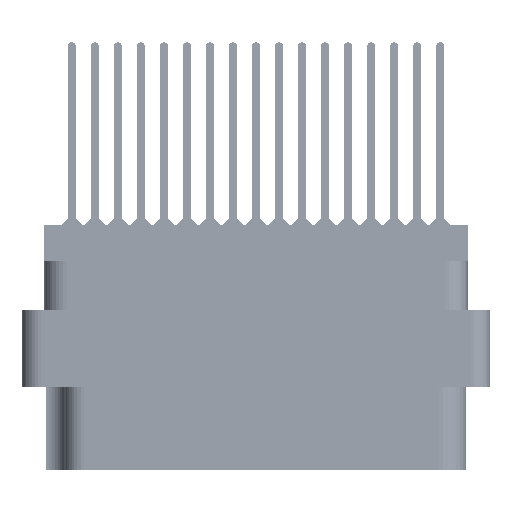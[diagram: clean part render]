
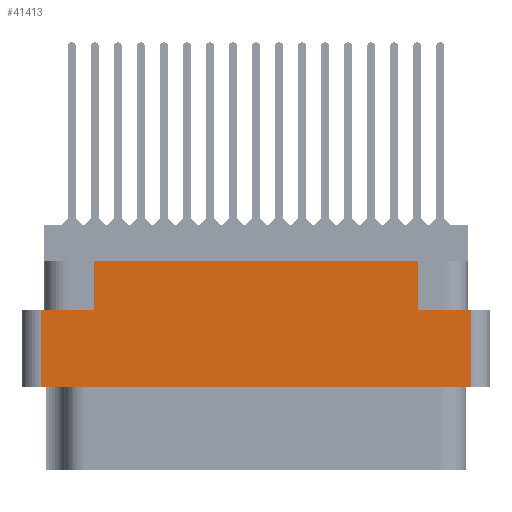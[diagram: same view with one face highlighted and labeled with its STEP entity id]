
A CAD part, left-side view. The second image highlights one B-rep face of the part: STEP entity #41413.
In plain terms, the highlighted planar face has unit normal (-1, 0, 0).
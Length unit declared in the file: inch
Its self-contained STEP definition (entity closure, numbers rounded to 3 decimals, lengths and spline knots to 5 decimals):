
#4939 = DIRECTION ( 'NONE',  ( 0., 0., 1. ) ) ;
#6147 = VECTOR ( 'NONE', #4939, 39.37008 ) ;
#7353 = DIRECTION ( 'NONE',  ( 0., -1., 0. ) ) ;
#7427 = CARTESIAN_POINT ( 'NONE',  ( -1.375, 0.7625, -0.117 ) ) ;
#7604 = CARTESIAN_POINT ( 'NONE',  ( -1.375, -0.7005, -0.798 ) ) ;
#7674 = CARTESIAN_POINT ( 'NONE',  ( -1.375, 0., -0.277 ) ) ;
#8654 = LINE ( 'NONE', #7604, #18909 ) ;
#11909 = VECTOR ( 'NONE', #84373, 39.37008 ) ;
#12399 = ORIENTED_EDGE ( 'NONE', *, *, #70454, .F. ) ;
#13224 = EDGE_CURVE ( 'NONE', #89813, #68162, #82296, .T. ) ;
#13752 = EDGE_CURVE ( 'NONE', #39072, #81822, #75394, .T. ) ;
#18715 = ORIENTED_EDGE ( 'NONE', *, *, #13752, .F. ) ;
#18909 = VECTOR ( 'NONE', #22811, 39.37008 ) ;
#20051 = LINE ( 'NONE', #7427, #66583 ) ;
#22471 = DIRECTION ( 'NONE',  ( 0., 0., 1. ) ) ;
#22811 = DIRECTION ( 'NONE',  ( 0., 0., 1. ) ) ;
#23578 = ORIENTED_EDGE ( 'NONE', *, *, #89172, .F. ) ;
#24195 = ORIENTED_EDGE ( 'NONE', *, *, #91789, .T. ) ;
#27021 = VERTEX_POINT ( 'NONE', #82789 ) ;
#27518 = CARTESIAN_POINT ( 'NONE',  ( -1.375, 0.5285, -0.117 ) ) ;
#28027 = DIRECTION ( 'NONE',  ( -1., 0., 0. ) ) ;
#29337 = LINE ( 'NONE', #7674, #58841 ) ;
#33437 = VECTOR ( 'NONE', #79629, 39.37008 ) ;
#35341 = ORIENTED_EDGE ( 'NONE', *, *, #47945, .F. ) ;
#38995 = AXIS2_PLACEMENT_3D ( 'NONE', #92511, #28027, #48742 ) ;
#39009 = VECTOR ( 'NONE', #22471, 39.37008 ) ;
#39072 = VERTEX_POINT ( 'NONE', #85633 ) ;
#40342 = EDGE_CURVE ( 'NONE', #90785, #66365, #8654, .T. ) ;
#41413 = ADVANCED_FACE ( 'NONE', ( #49441 ), #56936, .T. ) ;
#47945 = EDGE_CURVE ( 'NONE', #90785, #68162, #82249, .T. ) ;
#48142 = LINE ( 'NONE', #65962, #39009 ) ;
#48742 = DIRECTION ( 'NONE',  ( 0., 0., 1. ) ) ;
#49441 = FACE_OUTER_BOUND ( 'NONE', #58617, .T. ) ;
#50469 = CARTESIAN_POINT ( 'NONE',  ( -1.375, 0., -0.529 ) ) ;
#56936 = PLANE ( 'NONE',  #38995 ) ;
#57621 = DIRECTION ( 'NONE',  ( 0., -1., 0. ) ) ;
#58617 = EDGE_LOOP ( 'NONE', ( #12399, #67924, #35341, #63581, #23578, #24195, #81242, #18715 ) ) ;
#58841 = VECTOR ( 'NONE', #7353, 39.37008 ) ;
#60055 = VERTEX_POINT ( 'NONE', #82820 ) ;
#61854 = LINE ( 'NONE', #92574, #89124 ) ;
#63581 = ORIENTED_EDGE ( 'NONE', *, *, #40342, .T. ) ;
#65962 = CARTESIAN_POINT ( 'NONE',  ( -1.375, -0.5285, -0.277 ) ) ;
#66365 = VERTEX_POINT ( 'NONE', #68093 ) ;
#66583 = VECTOR ( 'NONE', #57621, 39.37008 ) ;
#67924 = ORIENTED_EDGE ( 'NONE', *, *, #13224, .T. ) ;
#68093 = CARTESIAN_POINT ( 'NONE',  ( -1.375, -0.7005, -0.277 ) ) ;
#68162 = VERTEX_POINT ( 'NONE', #82599 ) ;
#69620 = EDGE_CURVE ( 'NONE', #81822, #27021, #20051, .T. ) ;
#70257 = CARTESIAN_POINT ( 'NONE',  ( -1.375, -0.7005, -0.529 ) ) ;
#70454 = EDGE_CURVE ( 'NONE', #89813, #39072, #61854, .T. ) ;
#75394 = LINE ( 'NONE', #91957, #6147 ) ;
#77045 = CARTESIAN_POINT ( 'NONE',  ( -1.375, 0.7005, -0.798 ) ) ;
#79629 = DIRECTION ( 'NONE',  ( 0., 1., 0. ) ) ;
#81242 = ORIENTED_EDGE ( 'NONE', *, *, #69620, .F. ) ;
#81822 = VERTEX_POINT ( 'NONE', #27518 ) ;
#82249 = LINE ( 'NONE', #50469, #33437 ) ;
#82296 = LINE ( 'NONE', #77045, #11909 ) ;
#82599 = CARTESIAN_POINT ( 'NONE',  ( -1.375, 0.7005, -0.529 ) ) ;
#82789 = CARTESIAN_POINT ( 'NONE',  ( -1.375, -0.5285, -0.117 ) ) ;
#82820 = CARTESIAN_POINT ( 'NONE',  ( -1.375, -0.5285, -0.277 ) ) ;
#84373 = DIRECTION ( 'NONE',  ( 0., 0., -1. ) ) ;
#85633 = CARTESIAN_POINT ( 'NONE',  ( -1.375, 0.5285, -0.277 ) ) ;
#86944 = CARTESIAN_POINT ( 'NONE',  ( -1.375, 0.7005, -0.277 ) ) ;
#89124 = VECTOR ( 'NONE', #93842, 39.37008 ) ;
#89172 = EDGE_CURVE ( 'NONE', #60055, #66365, #29337, .T. ) ;
#89813 = VERTEX_POINT ( 'NONE', #86944 ) ;
#90785 = VERTEX_POINT ( 'NONE', #70257 ) ;
#91789 = EDGE_CURVE ( 'NONE', #60055, #27021, #48142, .T. ) ;
#91957 = CARTESIAN_POINT ( 'NONE',  ( -1.375, 0.5285, -0.277 ) ) ;
#92511 = CARTESIAN_POINT ( 'NONE',  ( -1.375, -0.7625, -0.798 ) ) ;
#92574 = CARTESIAN_POINT ( 'NONE',  ( -1.375, 0., -0.277 ) ) ;
#93842 = DIRECTION ( 'NONE',  ( 0., -1., 0. ) ) ;
